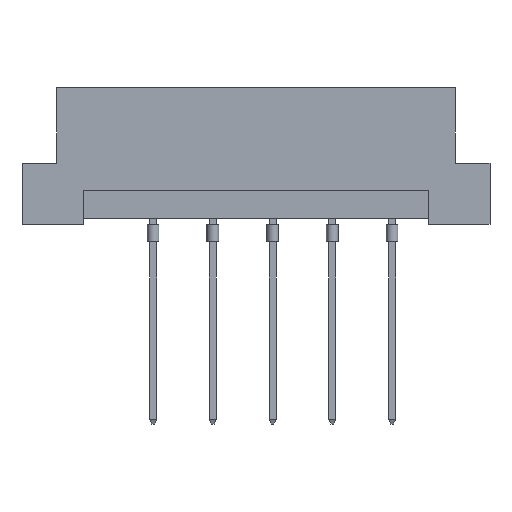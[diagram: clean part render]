
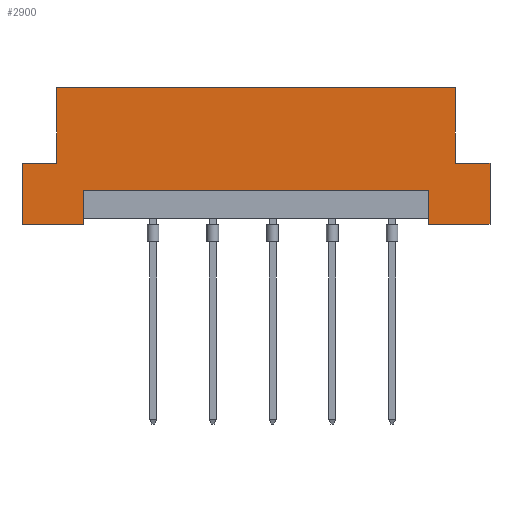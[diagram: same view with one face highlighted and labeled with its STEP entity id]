
A CAD part, front view. The second image highlights one B-rep face of the part: STEP entity #2900.
In plain terms, the highlighted planar face has unit normal (0, -1, 0).
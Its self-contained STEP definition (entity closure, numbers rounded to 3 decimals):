
#59 = DIRECTION ( 'NONE',  ( 0., 1., 0. ) ) ;
#77 = VECTOR ( 'NONE', #750, 1000. ) ;
#81 = CARTESIAN_POINT ( 'NONE',  ( 14.69, 0., 0. ) ) ;
#93 = PLANE ( 'NONE',  #2821 ) ;
#185 = CARTESIAN_POINT ( 'NONE',  ( -19.9, 0., 5.2 ) ) ;
#270 = CARTESIAN_POINT ( 'NONE',  ( 14.69, 0., 0.5 ) ) ;
#347 = ORIENTED_EDGE ( 'NONE', *, *, #2218, .F. ) ;
#384 = VECTOR ( 'NONE', #5717, 1000. ) ;
#447 = CARTESIAN_POINT ( 'NONE',  ( 14.69, 0., 2.9 ) ) ;
#449 = EDGE_CURVE ( 'NONE', #3725, #5126, #3310, .T. ) ;
#500 = EDGE_CURVE ( 'NONE', #1157, #5126, #2858, .T. ) ;
#537 = CARTESIAN_POINT ( 'NONE',  ( 19.9, 0., 5.2 ) ) ;
#624 = ORIENTED_EDGE ( 'NONE', *, *, #4105, .F. ) ;
#718 = VECTOR ( 'NONE', #4527, 1000. ) ;
#750 = DIRECTION ( 'NONE',  ( 0., 0., -1. ) ) ;
#764 = VERTEX_POINT ( 'NONE', #2841 ) ;
#873 = CARTESIAN_POINT ( 'NONE',  ( 16.94, 0., 5.2 ) ) ;
#888 = ORIENTED_EDGE ( 'NONE', *, *, #4928, .T. ) ;
#916 = CARTESIAN_POINT ( 'NONE',  ( 19.9, 0., 5.2 ) ) ;
#940 = LINE ( 'NONE', #2483, #718 ) ;
#1085 = CARTESIAN_POINT ( 'NONE',  ( -19.9, 0., 11.6 ) ) ;
#1121 = FACE_OUTER_BOUND ( 'NONE', #6344, .T. ) ;
#1143 = ORIENTED_EDGE ( 'NONE', *, *, #1546, .F. ) ;
#1157 = VERTEX_POINT ( 'NONE', #447 ) ;
#1416 = CARTESIAN_POINT ( 'NONE',  ( -14.69, 0., 0. ) ) ;
#1546 = EDGE_CURVE ( 'NONE', #1157, #764, #940, .T. ) ;
#1620 = EDGE_CURVE ( 'NONE', #1887, #5559, #4766, .T. ) ;
#1707 = VERTEX_POINT ( 'NONE', #5278 ) ;
#1779 = CARTESIAN_POINT ( 'NONE',  ( -16.94, 0., 5.2 ) ) ;
#1887 = VERTEX_POINT ( 'NONE', #873 ) ;
#1907 = CARTESIAN_POINT ( 'NONE',  ( -16.94, 0., 11.6 ) ) ;
#1935 = CARTESIAN_POINT ( 'NONE',  ( 16.94, 0., 5.2 ) ) ;
#2041 = CARTESIAN_POINT ( 'NONE',  ( -19.9, 0., 11.6 ) ) ;
#2170 = CARTESIAN_POINT ( 'NONE',  ( 19.9, 0., 0. ) ) ;
#2173 = VERTEX_POINT ( 'NONE', #5709 ) ;
#2218 = EDGE_CURVE ( 'NONE', #2173, #3518, #3840, .T. ) ;
#2269 = LINE ( 'NONE', #185, #6360 ) ;
#2364 = LINE ( 'NONE', #4503, #3919 ) ;
#2479 = ORIENTED_EDGE ( 'NONE', *, *, #3701, .F. ) ;
#2483 = CARTESIAN_POINT ( 'NONE',  ( 14.69, 0., 2.9 ) ) ;
#2634 = EDGE_CURVE ( 'NONE', #764, #3146, #4457, .T. ) ;
#2687 = LINE ( 'NONE', #4730, #4012 ) ;
#2722 = DIRECTION ( 'NONE',  ( 0., 0., 1. ) ) ;
#2790 = CARTESIAN_POINT ( 'NONE',  ( -19.9, 0., 0. ) ) ;
#2821 = AXIS2_PLACEMENT_3D ( 'NONE', #1085, #59, #4280 ) ;
#2841 = CARTESIAN_POINT ( 'NONE',  ( -14.69, 0., 2.9 ) ) ;
#2858 = LINE ( 'NONE', #270, #77 ) ;
#2895 = DIRECTION ( 'NONE',  ( 0., 0., -1. ) ) ;
#2900 = ADVANCED_FACE ( 'NONE', ( #1121 ), #93, .F. ) ;
#2944 = LINE ( 'NONE', #1935, #4290 ) ;
#3003 = EDGE_CURVE ( 'NONE', #5947, #3249, #2687, .T. ) ;
#3146 = VERTEX_POINT ( 'NONE', #1416 ) ;
#3249 = VERTEX_POINT ( 'NONE', #1907 ) ;
#3310 = LINE ( 'NONE', #2790, #4204 ) ;
#3518 = VERTEX_POINT ( 'NONE', #5339 ) ;
#3701 = EDGE_CURVE ( 'NONE', #3146, #2173, #6014, .T. ) ;
#3725 = VERTEX_POINT ( 'NONE', #2170 ) ;
#3840 = LINE ( 'NONE', #4270, #6044 ) ;
#3915 = VECTOR ( 'NONE', #5500, 1000. ) ;
#3919 = VECTOR ( 'NONE', #6555, 1000. ) ;
#4012 = VECTOR ( 'NONE', #2722, 1000. ) ;
#4105 = EDGE_CURVE ( 'NONE', #5559, #3725, #2364, .T. ) ;
#4204 = VECTOR ( 'NONE', #4873, 1000. ) ;
#4270 = CARTESIAN_POINT ( 'NONE',  ( -19.9, 0., 0. ) ) ;
#4280 = DIRECTION ( 'NONE',  ( 0., 0., 1. ) ) ;
#4290 = VECTOR ( 'NONE', #4544, 1000. ) ;
#4457 = LINE ( 'NONE', #5933, #4474 ) ;
#4474 = VECTOR ( 'NONE', #2895, 1000. ) ;
#4503 = CARTESIAN_POINT ( 'NONE',  ( 19.9, 0., 0. ) ) ;
#4527 = DIRECTION ( 'NONE',  ( -1., 0., 0. ) ) ;
#4544 = DIRECTION ( 'NONE',  ( 0., 0., 1. ) ) ;
#4615 = ORIENTED_EDGE ( 'NONE', *, *, #5244, .F. ) ;
#4730 = CARTESIAN_POINT ( 'NONE',  ( -16.94, 0., 5.2 ) ) ;
#4766 = LINE ( 'NONE', #537, #384 ) ;
#4873 = DIRECTION ( 'NONE',  ( -1., 0., 0. ) ) ;
#4928 = EDGE_CURVE ( 'NONE', #1887, #1707, #2944, .T. ) ;
#5060 = CARTESIAN_POINT ( 'NONE',  ( -19.9, 0., 0. ) ) ;
#5064 = VECTOR ( 'NONE', #5176, 1000. ) ;
#5126 = VERTEX_POINT ( 'NONE', #81 ) ;
#5176 = DIRECTION ( 'NONE',  ( 1., 0., 0. ) ) ;
#5210 = LINE ( 'NONE', #2041, #5064 ) ;
#5244 = EDGE_CURVE ( 'NONE', #3518, #5947, #2269, .T. ) ;
#5259 = ORIENTED_EDGE ( 'NONE', *, *, #2634, .F. ) ;
#5278 = CARTESIAN_POINT ( 'NONE',  ( 16.94, 0., 11.6 ) ) ;
#5336 = DIRECTION ( 'NONE',  ( 0., 0., 1. ) ) ;
#5339 = CARTESIAN_POINT ( 'NONE',  ( -19.9, 0., 5.2 ) ) ;
#5495 = ORIENTED_EDGE ( 'NONE', *, *, #1620, .F. ) ;
#5500 = DIRECTION ( 'NONE',  ( -1., 0., 0. ) ) ;
#5559 = VERTEX_POINT ( 'NONE', #916 ) ;
#5709 = CARTESIAN_POINT ( 'NONE',  ( -19.9, 0., 0. ) ) ;
#5717 = DIRECTION ( 'NONE',  ( 1., 0., 0. ) ) ;
#5824 = EDGE_CURVE ( 'NONE', #3249, #1707, #5210, .T. ) ;
#5933 = CARTESIAN_POINT ( 'NONE',  ( -14.69, 0., 0.5 ) ) ;
#5943 = DIRECTION ( 'NONE',  ( 1., 0., 0. ) ) ;
#5947 = VERTEX_POINT ( 'NONE', #1779 ) ;
#6014 = LINE ( 'NONE', #5060, #3915 ) ;
#6037 = ORIENTED_EDGE ( 'NONE', *, *, #5824, .F. ) ;
#6044 = VECTOR ( 'NONE', #5336, 1000. ) ;
#6344 = EDGE_LOOP ( 'NONE', ( #1143, #6519, #6692, #624, #5495, #888, #6037, #6604, #4615, #347, #2479, #5259 ) ) ;
#6360 = VECTOR ( 'NONE', #5943, 1000. ) ;
#6519 = ORIENTED_EDGE ( 'NONE', *, *, #500, .T. ) ;
#6555 = DIRECTION ( 'NONE',  ( 0., 0., -1. ) ) ;
#6604 = ORIENTED_EDGE ( 'NONE', *, *, #3003, .F. ) ;
#6692 = ORIENTED_EDGE ( 'NONE', *, *, #449, .F. ) ;
